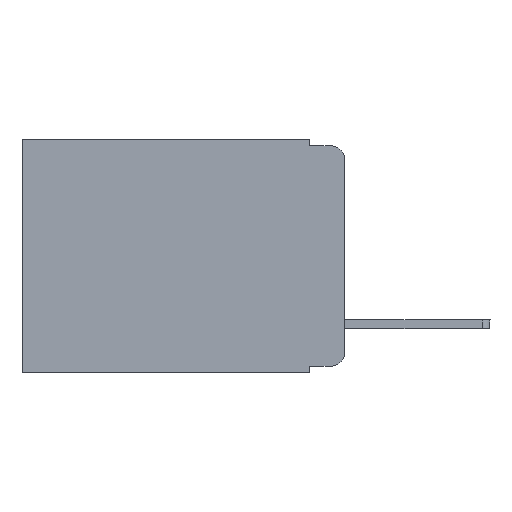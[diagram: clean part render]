
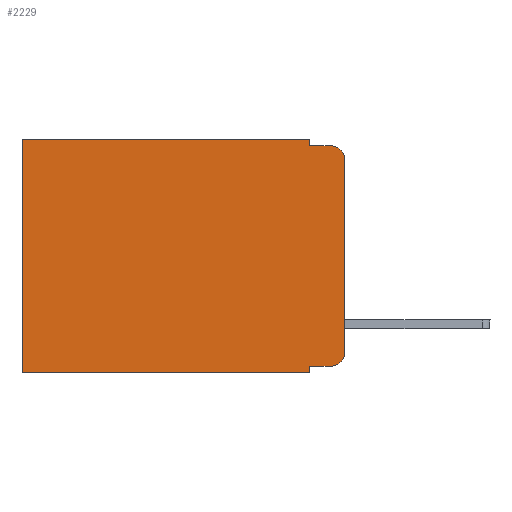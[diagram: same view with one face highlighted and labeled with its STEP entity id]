
A CAD part, left-side view. The second image highlights one B-rep face of the part: STEP entity #2229.
In plain terms, the highlighted planar face has unit normal (-1, 0, 0).
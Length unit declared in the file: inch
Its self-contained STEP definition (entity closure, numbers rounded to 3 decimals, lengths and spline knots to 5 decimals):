
#213 = EDGE_CURVE ( 'NONE', #10662, #7963, #10190, .T. ) ;
#285 = EDGE_CURVE ( 'NONE', #10662, #5021, #8625, .T. ) ;
#321 = CARTESIAN_POINT ( 'NONE',  ( 0.298, 0.473, 0. ) ) ;
#622 = CARTESIAN_POINT ( 'NONE',  ( 0.298, 0., -0.343 ) ) ;
#834 = VECTOR ( 'NONE', #10256, 39.37008 ) ;
#852 = CARTESIAN_POINT ( 'NONE',  ( 0.298, 0.051, -0.333 ) ) ;
#971 = CARTESIAN_POINT ( 'NONE',  ( 0.298, 0.02, -0.03 ) ) ;
#1375 = DIRECTION ( 'NONE',  ( 0., 1., 0. ) ) ;
#1499 = EDGE_CURVE ( 'NONE', #2323, #8835, #6673, .T. ) ;
#1583 = CARTESIAN_POINT ( 'NONE',  ( 0.298, 0.051, 0. ) ) ;
#1636 = VERTEX_POINT ( 'NONE', #9776 ) ;
#1968 = ORIENTED_EDGE ( 'NONE', *, *, #285, .T. ) ;
#2051 = EDGE_CURVE ( 'NONE', #8835, #1636, #10630, .T. ) ;
#2229 = ADVANCED_FACE ( 'NONE', ( #10342 ), #6878, .F. ) ;
#2295 = CARTESIAN_POINT ( 'NONE',  ( 0.298, 0.473, 0. ) ) ;
#2323 = VERTEX_POINT ( 'NONE', #1583 ) ;
#2696 = CARTESIAN_POINT ( 'NONE',  ( 0.298, 0.051, -0.01 ) ) ;
#2703 = CARTESIAN_POINT ( 'NONE',  ( 0.298, 0.051, -0.343 ) ) ;
#2726 = LINE ( 'NONE', #8923, #8240 ) ;
#2735 = DIRECTION ( 'NONE',  ( 0., 0., -1. ) ) ;
#2813 = EDGE_CURVE ( 'NONE', #7963, #9553, #9330, .T. ) ;
#3083 = VECTOR ( 'NONE', #7941, 39.37008 ) ;
#3112 = CARTESIAN_POINT ( 'NONE',  ( 0.298, 0.051, 0. ) ) ;
#3220 = EDGE_CURVE ( 'NONE', #5021, #5892, #10654, .T. ) ;
#3420 = LINE ( 'NONE', #4470, #3083 ) ;
#3484 = CARTESIAN_POINT ( 'NONE',  ( 0.298, 0.051, -0.01 ) ) ;
#3508 = ORIENTED_EDGE ( 'NONE', *, *, #213, .F. ) ;
#4078 = EDGE_LOOP ( 'NONE', ( #10327, #11282, #5287, #8943, #5708, #5719, #9449, #3508, #1968, #4950 ) ) ;
#4329 = DIRECTION ( 'NONE',  ( -1., 0., 0. ) ) ;
#4388 = VERTEX_POINT ( 'NONE', #8518 ) ;
#4470 = CARTESIAN_POINT ( 'NONE',  ( 0.298, 0., 0. ) ) ;
#4537 = DIRECTION ( 'NONE',  ( -1., 0., 0. ) ) ;
#4950 = ORIENTED_EDGE ( 'NONE', *, *, #3220, .T. ) ;
#5017 = DIRECTION ( 'NONE',  ( 0., 0., -1. ) ) ;
#5021 = VERTEX_POINT ( 'NONE', #6458 ) ;
#5076 = CARTESIAN_POINT ( 'NONE',  ( 0.298, 0., 0. ) ) ;
#5082 = VECTOR ( 'NONE', #5685, 39.37008 ) ;
#5287 = ORIENTED_EDGE ( 'NONE', *, *, #2051, .F. ) ;
#5437 = DIRECTION ( 'NONE',  ( 0., -1., 0. ) ) ;
#5464 = CARTESIAN_POINT ( 'NONE',  ( 0.298, 0., -0.313 ) ) ;
#5685 = DIRECTION ( 'NONE',  ( 0., 0., -1. ) ) ;
#5708 = ORIENTED_EDGE ( 'NONE', *, *, #10609, .T. ) ;
#5719 = ORIENTED_EDGE ( 'NONE', *, *, #6059, .T. ) ;
#5728 = DIRECTION ( 'NONE',  ( 0., 0., -1. ) ) ;
#5738 = AXIS2_PLACEMENT_3D ( 'NONE', #971, #4537, #2735 ) ;
#5763 = EDGE_CURVE ( 'NONE', #4388, #5892, #2726, .T. ) ;
#5828 = VECTOR ( 'NONE', #5437, 39.37008 ) ;
#5892 = VERTEX_POINT ( 'NONE', #5464 ) ;
#6059 = EDGE_CURVE ( 'NONE', #7874, #9553, #8284, .T. ) ;
#6458 = CARTESIAN_POINT ( 'NONE',  ( 0.298, 0.02, -0.333 ) ) ;
#6673 = LINE ( 'NONE', #10029, #5082 ) ;
#6741 = VECTOR ( 'NONE', #6791, 39.37008 ) ;
#6791 = DIRECTION ( 'NONE',  ( 0., -1., 0. ) ) ;
#6878 = PLANE ( 'NONE',  #11007 ) ;
#7080 = DIRECTION ( 'NONE',  ( 0., 0., -1. ) ) ;
#7874 = VERTEX_POINT ( 'NONE', #2295 ) ;
#7941 = DIRECTION ( 'NONE',  ( 0., 1., 0. ) ) ;
#7963 = VERTEX_POINT ( 'NONE', #2703 ) ;
#8240 = VECTOR ( 'NONE', #7080, 39.37008 ) ;
#8266 = CARTESIAN_POINT ( 'NONE',  ( 0.298, 0.473, -0.343 ) ) ;
#8284 = LINE ( 'NONE', #321, #834 ) ;
#8451 = CARTESIAN_POINT ( 'NONE',  ( 0.298, 0.051, -0.333 ) ) ;
#8483 = DIRECTION ( 'NONE',  ( 1., 0., 0. ) ) ;
#8518 = CARTESIAN_POINT ( 'NONE',  ( 0.298, 0., -0.03 ) ) ;
#8625 = LINE ( 'NONE', #8451, #6741 ) ;
#8814 = AXIS2_PLACEMENT_3D ( 'NONE', #11329, #4329, #11157 ) ;
#8835 = VERTEX_POINT ( 'NONE', #3484 ) ;
#8923 = CARTESIAN_POINT ( 'NONE',  ( 0.298, 0., 0. ) ) ;
#8943 = ORIENTED_EDGE ( 'NONE', *, *, #1499, .F. ) ;
#9059 = EDGE_CURVE ( 'NONE', #4388, #1636, #11274, .T. ) ;
#9330 = LINE ( 'NONE', #622, #9545 ) ;
#9449 = ORIENTED_EDGE ( 'NONE', *, *, #2813, .F. ) ;
#9545 = VECTOR ( 'NONE', #1375, 39.37008 ) ;
#9553 = VERTEX_POINT ( 'NONE', #8266 ) ;
#9672 = VECTOR ( 'NONE', #5728, 39.37008 ) ;
#9776 = CARTESIAN_POINT ( 'NONE',  ( 0.298, 0.02, -0.01 ) ) ;
#10029 = CARTESIAN_POINT ( 'NONE',  ( 0.298, 0.051, 0. ) ) ;
#10190 = LINE ( 'NONE', #3112, #9672 ) ;
#10256 = DIRECTION ( 'NONE',  ( 0., 0., -1. ) ) ;
#10327 = ORIENTED_EDGE ( 'NONE', *, *, #5763, .F. ) ;
#10342 = FACE_OUTER_BOUND ( 'NONE', #4078, .T. ) ;
#10609 = EDGE_CURVE ( 'NONE', #2323, #7874, #3420, .T. ) ;
#10630 = LINE ( 'NONE', #2696, #5828 ) ;
#10654 = CIRCLE ( 'NONE', #8814, 0.02 ) ;
#10662 = VERTEX_POINT ( 'NONE', #852 ) ;
#11007 = AXIS2_PLACEMENT_3D ( 'NONE', #5076, #8483, #5017 ) ;
#11157 = DIRECTION ( 'NONE',  ( 0., 0., -1. ) ) ;
#11274 = CIRCLE ( 'NONE', #5738, 0.02 ) ;
#11282 = ORIENTED_EDGE ( 'NONE', *, *, #9059, .T. ) ;
#11329 = CARTESIAN_POINT ( 'NONE',  ( 0.298, 0.02, -0.313 ) ) ;
